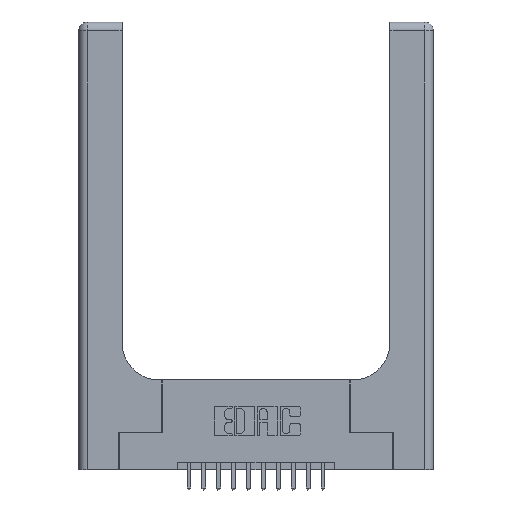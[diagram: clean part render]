
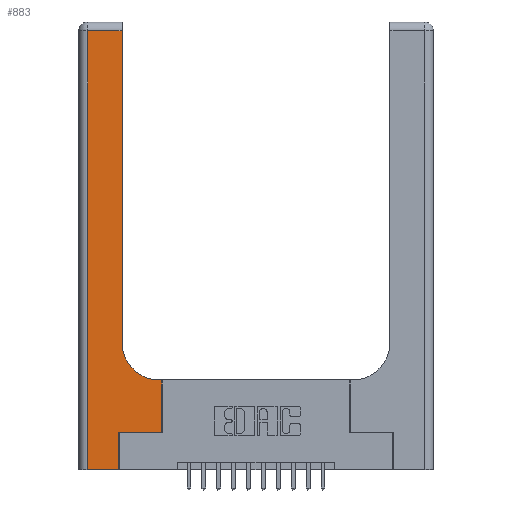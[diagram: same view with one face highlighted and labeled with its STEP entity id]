
A CAD part, top view. The second image highlights one B-rep face of the part: STEP entity #883.
In plain terms, the highlighted planar face has unit normal (0, 0, 1).
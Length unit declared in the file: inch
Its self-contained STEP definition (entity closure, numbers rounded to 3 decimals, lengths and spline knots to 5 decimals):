
#258 = LINE ( 'NONE', #11568, #10114 ) ;
#555 = EDGE_CURVE ( 'NONE', #8823, #5233, #258, .T. ) ;
#819 = VECTOR ( 'NONE', #12326, 39.37008 ) ;
#883 = ADVANCED_FACE ( 'NONE', ( #12158 ), #1794, .F. ) ;
#1061 = DIRECTION ( 'NONE',  ( 0., 0., -1. ) ) ;
#1205 = ORIENTED_EDGE ( 'NONE', *, *, #9868, .T. ) ;
#1275 = VERTEX_POINT ( 'NONE', #10603 ) ;
#1628 = CARTESIAN_POINT ( 'NONE',  ( 0.2915, 3., 0.37 ) ) ;
#1721 = ORIENTED_EDGE ( 'NONE', *, *, #3385, .T. ) ;
#1794 = PLANE ( 'NONE',  #15381 ) ;
#1796 = LINE ( 'NONE', #15962, #13495 ) ;
#2015 = LINE ( 'NONE', #11681, #15818 ) ;
#2356 = CARTESIAN_POINT ( 'NONE',  ( 0., 3., 0.37 ) ) ;
#2418 = DIRECTION ( 'NONE',  ( -1., 0., 0. ) ) ;
#2635 = AXIS2_PLACEMENT_3D ( 'NONE', #6261, #11511, #15560 ) ;
#2954 = ORIENTED_EDGE ( 'NONE', *, *, #13321, .T. ) ;
#3385 = EDGE_CURVE ( 'NONE', #16286, #4690, #2015, .T. ) ;
#4042 = DIRECTION ( 'NONE',  ( -1., 0., 0. ) ) ;
#4169 = EDGE_CURVE ( 'NONE', #1275, #6883, #1796, .T. ) ;
#4690 = VERTEX_POINT ( 'NONE', #12876 ) ;
#5140 = CARTESIAN_POINT ( 'NONE',  ( 0.5585, 0.6, 0.37 ) ) ;
#5233 = VERTEX_POINT ( 'NONE', #12880 ) ;
#5377 = CARTESIAN_POINT ( 'NONE',  ( 0.06, 0., 0.37 ) ) ;
#6014 = VERTEX_POINT ( 'NONE', #13877 ) ;
#6171 = VECTOR ( 'NONE', #8358, 39.37008 ) ;
#6230 = CARTESIAN_POINT ( 'NONE',  ( 0.06, 2.94, 0.37 ) ) ;
#6261 = CARTESIAN_POINT ( 'NONE',  ( 0.5415, 0.85, 0.37 ) ) ;
#6652 = CARTESIAN_POINT ( 'NONE',  ( 0.269, 0., 0.37 ) ) ;
#6758 = EDGE_CURVE ( 'NONE', #11269, #1275, #16554, .T. ) ;
#6883 = VERTEX_POINT ( 'NONE', #6230 ) ;
#7179 = CARTESIAN_POINT ( 'NONE',  ( 0.06, 3., 0.37 ) ) ;
#7240 = LINE ( 'NONE', #14948, #8505 ) ;
#7275 = CIRCLE ( 'NONE', #2635, 0.25 ) ;
#7431 = LINE ( 'NONE', #7179, #6171 ) ;
#7723 = ORIENTED_EDGE ( 'NONE', *, *, #6758, .T. ) ;
#7997 = ORIENTED_EDGE ( 'NONE', *, *, #10915, .T. ) ;
#8358 = DIRECTION ( 'NONE',  ( 0., -1., 0. ) ) ;
#8505 = VECTOR ( 'NONE', #12312, 39.37008 ) ;
#8774 = ORIENTED_EDGE ( 'NONE', *, *, #12521, .T. ) ;
#8823 = VERTEX_POINT ( 'NONE', #5377 ) ;
#8897 = DIRECTION ( 'NONE',  ( 1., 0., 0. ) ) ;
#9493 = VECTOR ( 'NONE', #9692, 39.37008 ) ;
#9692 = DIRECTION ( 'NONE',  ( -1., 0., 0. ) ) ;
#9868 = EDGE_CURVE ( 'NONE', #6014, #11269, #7275, .T. ) ;
#9887 = LINE ( 'NONE', #12527, #9493 ) ;
#10114 = VECTOR ( 'NONE', #8897, 39.37008 ) ;
#10476 = ORIENTED_EDGE ( 'NONE', *, *, #11776, .T. ) ;
#10537 = LINE ( 'NONE', #6652, #10947 ) ;
#10603 = CARTESIAN_POINT ( 'NONE',  ( 0.2915, 2.94, 0.37 ) ) ;
#10915 = EDGE_CURVE ( 'NONE', #4690, #12611, #7240, .T. ) ;
#10947 = VECTOR ( 'NONE', #16272, 39.37008 ) ;
#11269 = VERTEX_POINT ( 'NONE', #15520 ) ;
#11511 = DIRECTION ( 'NONE',  ( 0., 0., -1. ) ) ;
#11568 = CARTESIAN_POINT ( 'NONE',  ( 0., 0., 0.37 ) ) ;
#11681 = CARTESIAN_POINT ( 'NONE',  ( 0.269, 0.25, 0.37 ) ) ;
#11776 = EDGE_CURVE ( 'NONE', #5233, #16286, #10537, .T. ) ;
#12158 = FACE_OUTER_BOUND ( 'NONE', #14370, .T. ) ;
#12312 = DIRECTION ( 'NONE',  ( 0., 1., 0. ) ) ;
#12326 = DIRECTION ( 'NONE',  ( 0., 1., 0. ) ) ;
#12521 = EDGE_CURVE ( 'NONE', #6883, #8823, #7431, .T. ) ;
#12527 = CARTESIAN_POINT ( 'NONE',  ( 0.2915, 0.6, 0.37 ) ) ;
#12611 = VERTEX_POINT ( 'NONE', #5140 ) ;
#12876 = CARTESIAN_POINT ( 'NONE',  ( 0.5585, 0.25, 0.37 ) ) ;
#12880 = CARTESIAN_POINT ( 'NONE',  ( 0.269, 0., 0.37 ) ) ;
#13321 = EDGE_CURVE ( 'NONE', #12611, #6014, #9887, .T. ) ;
#13495 = VECTOR ( 'NONE', #4042, 39.37008 ) ;
#13877 = CARTESIAN_POINT ( 'NONE',  ( 0.5415, 0.6, 0.37 ) ) ;
#14335 = CARTESIAN_POINT ( 'NONE',  ( 0.269, 0.25, 0.37 ) ) ;
#14370 = EDGE_LOOP ( 'NONE', ( #7723, #14616, #8774, #16843, #10476, #1721, #7997, #2954, #1205 ) ) ;
#14616 = ORIENTED_EDGE ( 'NONE', *, *, #4169, .T. ) ;
#14948 = CARTESIAN_POINT ( 'NONE',  ( 0.5585, 0.25, 0.37 ) ) ;
#15381 = AXIS2_PLACEMENT_3D ( 'NONE', #2356, #1061, #2418 ) ;
#15520 = CARTESIAN_POINT ( 'NONE',  ( 0.2915, 0.85, 0.37 ) ) ;
#15560 = DIRECTION ( 'NONE',  ( 1., 0., 0. ) ) ;
#15818 = VECTOR ( 'NONE', #15910, 39.37008 ) ;
#15910 = DIRECTION ( 'NONE',  ( 1., 0., 0. ) ) ;
#15962 = CARTESIAN_POINT ( 'NONE',  ( 0., 2.94, 0.37 ) ) ;
#16272 = DIRECTION ( 'NONE',  ( 0., 1., 0. ) ) ;
#16286 = VERTEX_POINT ( 'NONE', #14335 ) ;
#16554 = LINE ( 'NONE', #1628, #819 ) ;
#16843 = ORIENTED_EDGE ( 'NONE', *, *, #555, .T. ) ;
